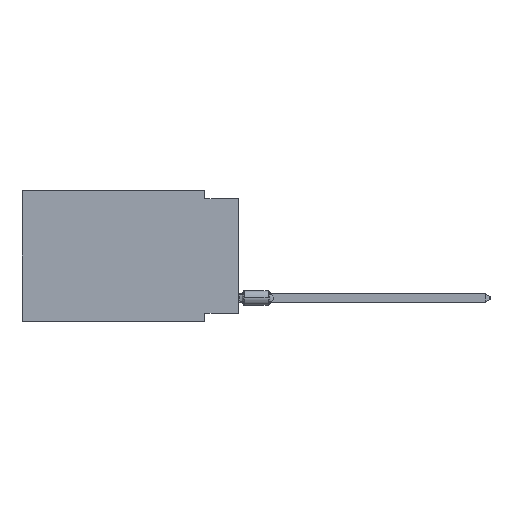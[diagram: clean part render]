
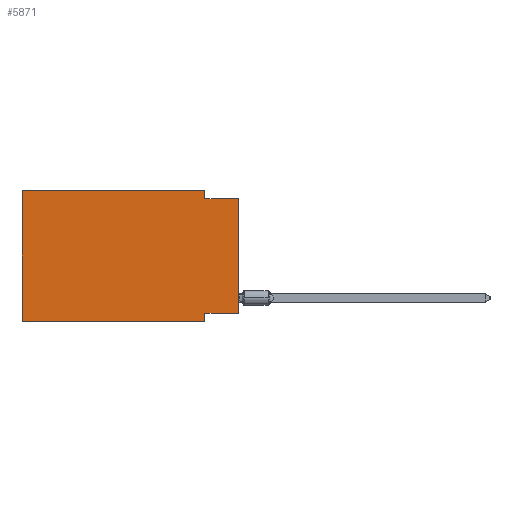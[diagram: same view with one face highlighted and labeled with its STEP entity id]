
A CAD part, left-side view. The second image highlights one B-rep face of the part: STEP entity #5871.
In plain terms, the highlighted planar face has unit normal (-1, 0, 0).
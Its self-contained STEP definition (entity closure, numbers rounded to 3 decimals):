
#37 = CARTESIAN_POINT ( 'NONE',  ( 0., 0., -9.271 ) ) ;
#1226 = DIRECTION ( 'NONE',  ( 0., -1., 0. ) ) ;
#1238 = CARTESIAN_POINT ( 'NONE',  ( 0., 2.54, 0. ) ) ;
#1355 = DIRECTION ( 'NONE',  ( 0., 0., 1. ) ) ;
#2452 = CARTESIAN_POINT ( 'NONE',  ( 0., 16.383, 0. ) ) ;
#2631 = EDGE_CURVE ( 'NONE', #46633, #20913, #15817, .T. ) ;
#2998 = VERTEX_POINT ( 'NONE', #20882 ) ;
#4567 = ORIENTED_EDGE ( 'NONE', *, *, #17489, .F. ) ;
#4679 = LINE ( 'NONE', #5325, #10063 ) ;
#5325 = CARTESIAN_POINT ( 'NONE',  ( 0., 16.383, -9.906 ) ) ;
#5871 = ADVANCED_FACE ( 'NONE', ( #21322 ), #40867, .F. ) ;
#7472 = VECTOR ( 'NONE', #19016, 1000. ) ;
#8367 = ORIENTED_EDGE ( 'NONE', *, *, #2631, .T. ) ;
#9913 = LINE ( 'NONE', #1238, #50143 ) ;
#10063 = VECTOR ( 'NONE', #18838, 1000. ) ;
#11506 = VERTEX_POINT ( 'NONE', #23640 ) ;
#11889 = EDGE_LOOP ( 'NONE', ( #8367, #4567, #39534, #18530, #58393, #57563, #32201, #39436 ) ) ;
#12505 = CARTESIAN_POINT ( 'NONE',  ( 0., 0., -9.271 ) ) ;
#12667 = VERTEX_POINT ( 'NONE', #59361 ) ;
#15817 = LINE ( 'NONE', #39859, #22636 ) ;
#16122 = DIRECTION ( 'NONE',  ( 0., 0., 1. ) ) ;
#17489 = EDGE_CURVE ( 'NONE', #2998, #20913, #18057, .T. ) ;
#18057 = LINE ( 'NONE', #28337, #7472 ) ;
#18530 = ORIENTED_EDGE ( 'NONE', *, *, #52535, .F. ) ;
#18838 = DIRECTION ( 'NONE',  ( 0., -1., 0. ) ) ;
#19016 = DIRECTION ( 'NONE',  ( 0., -1., 0. ) ) ;
#20618 = VECTOR ( 'NONE', #1226, 1000. ) ;
#20882 = CARTESIAN_POINT ( 'NONE',  ( 0., 2.54, -0.635 ) ) ;
#20913 = VERTEX_POINT ( 'NONE', #60205 ) ;
#21137 = LINE ( 'NONE', #60251, #20618 ) ;
#21322 = FACE_OUTER_BOUND ( 'NONE', #11889, .T. ) ;
#22636 = VECTOR ( 'NONE', #16122, 1000. ) ;
#22959 = VERTEX_POINT ( 'NONE', #26057 ) ;
#23640 = CARTESIAN_POINT ( 'NONE',  ( 0., 2.54, 0. ) ) ;
#24129 = EDGE_CURVE ( 'NONE', #11506, #2998, #9913, .T. ) ;
#25465 = VECTOR ( 'NONE', #52632, 1000. ) ;
#26057 = CARTESIAN_POINT ( 'NONE',  ( 0., 16.383, -9.906 ) ) ;
#27380 = DIRECTION ( 'NONE',  ( 1., 0., 0. ) ) ;
#28337 = CARTESIAN_POINT ( 'NONE',  ( 0., 0., -0.635 ) ) ;
#28573 = CARTESIAN_POINT ( 'NONE',  ( 0., 2.54, -9.906 ) ) ;
#28655 = EDGE_CURVE ( 'NONE', #46633, #28784, #59079, .T. ) ;
#28784 = VERTEX_POINT ( 'NONE', #59403 ) ;
#30542 = DIRECTION ( 'NONE',  ( 0., 1., 0. ) ) ;
#31343 = VECTOR ( 'NONE', #1355, 1000. ) ;
#32191 = DIRECTION ( 'NONE',  ( 0., 0., -1. ) ) ;
#32201 = ORIENTED_EDGE ( 'NONE', *, *, #55153, .F. ) ;
#35508 = EDGE_CURVE ( 'NONE', #22959, #12667, #4679, .T. ) ;
#37921 = VERTEX_POINT ( 'NONE', #2452 ) ;
#39436 = ORIENTED_EDGE ( 'NONE', *, *, #28655, .F. ) ;
#39534 = ORIENTED_EDGE ( 'NONE', *, *, #24129, .F. ) ;
#39859 = CARTESIAN_POINT ( 'NONE',  ( 0., 0., 0. ) ) ;
#40867 = PLANE ( 'NONE',  #47448 ) ;
#41133 = LINE ( 'NONE', #45624, #31343 ) ;
#45063 = EDGE_CURVE ( 'NONE', #22959, #37921, #41133, .T. ) ;
#45624 = CARTESIAN_POINT ( 'NONE',  ( 0., 16.383, 0. ) ) ;
#46633 = VERTEX_POINT ( 'NONE', #12505 ) ;
#47448 = AXIS2_PLACEMENT_3D ( 'NONE', #49235, #27380, #32191 ) ;
#49235 = CARTESIAN_POINT ( 'NONE',  ( 0., 16.383, 0. ) ) ;
#50143 = VECTOR ( 'NONE', #58999, 1000. ) ;
#52535 = EDGE_CURVE ( 'NONE', #37921, #11506, #21137, .T. ) ;
#52632 = DIRECTION ( 'NONE',  ( 0., 0., -1. ) ) ;
#55153 = EDGE_CURVE ( 'NONE', #28784, #12667, #62240, .T. ) ;
#56538 = VECTOR ( 'NONE', #30542, 1000. ) ;
#57563 = ORIENTED_EDGE ( 'NONE', *, *, #35508, .T. ) ;
#58393 = ORIENTED_EDGE ( 'NONE', *, *, #45063, .F. ) ;
#58999 = DIRECTION ( 'NONE',  ( 0., 0., -1. ) ) ;
#59079 = LINE ( 'NONE', #37, #56538 ) ;
#59361 = CARTESIAN_POINT ( 'NONE',  ( 0., 2.54, -9.906 ) ) ;
#59403 = CARTESIAN_POINT ( 'NONE',  ( 0., 2.54, -9.271 ) ) ;
#60205 = CARTESIAN_POINT ( 'NONE',  ( 0., 0., -0.635 ) ) ;
#60251 = CARTESIAN_POINT ( 'NONE',  ( 0., 16.383, 0. ) ) ;
#62240 = LINE ( 'NONE', #28573, #25465 ) ;
